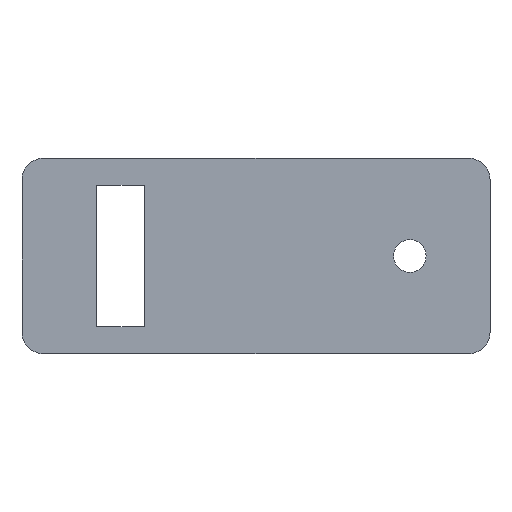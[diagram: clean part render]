
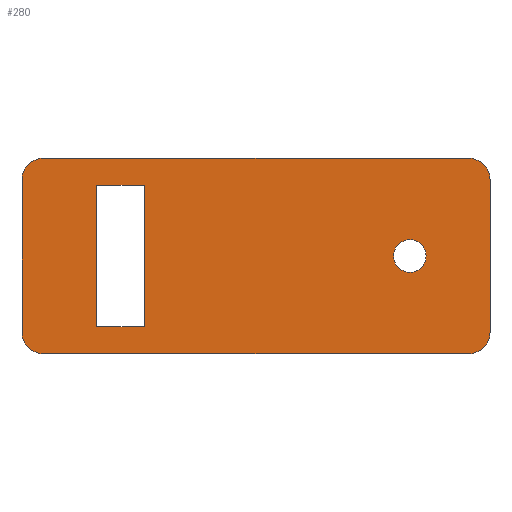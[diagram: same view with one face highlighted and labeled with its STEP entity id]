
A CAD part, top view. The second image highlights one B-rep face of the part: STEP entity #280.
In plain terms, the highlighted planar face has unit normal (0, 0, 1).
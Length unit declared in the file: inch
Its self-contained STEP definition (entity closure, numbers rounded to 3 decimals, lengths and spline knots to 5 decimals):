
#15=FACE_BOUND('',#46,.T.);
#16=FACE_BOUND('',#47,.T.);
#19=PLANE('',#311);
#30=FACE_OUTER_BOUND('',#45,.T.);
#45=EDGE_LOOP('',(#200,#201,#202,#203,#204,#205,#206,#207));
#46=EDGE_LOOP('',(#208,#209,#210,#211));
#47=EDGE_LOOP('',(#212));
#65=LINE('',#426,#94);
#66=LINE('',#430,#95);
#67=LINE('',#434,#96);
#68=LINE('',#437,#97);
#69=LINE('',#440,#98);
#70=LINE('',#442,#99);
#71=LINE('',#444,#100);
#72=LINE('',#445,#101);
#94=VECTOR('',#345,0.3937);
#95=VECTOR('',#348,0.3937);
#96=VECTOR('',#351,0.3937);
#97=VECTOR('',#354,0.3937);
#98=VECTOR('',#355,0.3937);
#99=VECTOR('',#356,0.3937);
#100=VECTOR('',#357,0.3937);
#101=VECTOR('',#358,0.3937);
#121=CIRCLE('',#309,0.11811);
#123=CIRCLE('',#312,0.11811);
#124=CIRCLE('',#313,0.11811);
#125=CIRCLE('',#314,0.11811);
#126=CIRCLE('',#315,0.0885);
#131=VERTEX_POINT('',#416);
#132=VERTEX_POINT('',#417);
#135=VERTEX_POINT('',#425);
#136=VERTEX_POINT('',#427);
#137=VERTEX_POINT('',#429);
#138=VERTEX_POINT('',#431);
#139=VERTEX_POINT('',#433);
#140=VERTEX_POINT('',#435);
#141=VERTEX_POINT('',#438);
#142=VERTEX_POINT('',#439);
#143=VERTEX_POINT('',#441);
#144=VERTEX_POINT('',#443);
#145=VERTEX_POINT('',#446);
#157=EDGE_CURVE('',#131,#132,#121,.T.);
#161=EDGE_CURVE('',#131,#135,#65,.T.);
#162=EDGE_CURVE('',#136,#135,#123,.T.);
#163=EDGE_CURVE('',#137,#136,#66,.T.);
#164=EDGE_CURVE('',#138,#137,#124,.T.);
#165=EDGE_CURVE('',#138,#139,#67,.T.);
#166=EDGE_CURVE('',#140,#139,#125,.T.);
#167=EDGE_CURVE('',#132,#140,#68,.T.);
#168=EDGE_CURVE('',#141,#142,#69,.T.);
#169=EDGE_CURVE('',#143,#141,#70,.T.);
#170=EDGE_CURVE('',#144,#143,#71,.T.);
#171=EDGE_CURVE('',#142,#144,#72,.T.);
#172=EDGE_CURVE('',#145,#145,#126,.T.);
#200=ORIENTED_EDGE('',*,*,#157,.F.);
#201=ORIENTED_EDGE('',*,*,#161,.T.);
#202=ORIENTED_EDGE('',*,*,#162,.F.);
#203=ORIENTED_EDGE('',*,*,#163,.F.);
#204=ORIENTED_EDGE('',*,*,#164,.F.);
#205=ORIENTED_EDGE('',*,*,#165,.T.);
#206=ORIENTED_EDGE('',*,*,#166,.F.);
#207=ORIENTED_EDGE('',*,*,#167,.F.);
#208=ORIENTED_EDGE('',*,*,#168,.F.);
#209=ORIENTED_EDGE('',*,*,#169,.F.);
#210=ORIENTED_EDGE('',*,*,#170,.F.);
#211=ORIENTED_EDGE('',*,*,#171,.F.);
#212=ORIENTED_EDGE('',*,*,#172,.F.);
#280=ADVANCED_FACE('',(#30,#15,#16),#19,.F.);
#309=AXIS2_PLACEMENT_3D('',#418,#337,#338);
#311=AXIS2_PLACEMENT_3D('',#424,#343,#344);
#312=AXIS2_PLACEMENT_3D('',#428,#346,#347);
#313=AXIS2_PLACEMENT_3D('',#432,#349,#350);
#314=AXIS2_PLACEMENT_3D('',#436,#352,#353);
#315=AXIS2_PLACEMENT_3D('',#447,#359,#360);
#337=DIRECTION('center_axis',(0.,0.,
-1.));
#338=DIRECTION('ref_axis',(-0.707,0.707,0.));
#343=DIRECTION('center_axis',(0.,0.,
-1.));
#344=DIRECTION('ref_axis',(1.,0.,0.));
#345=DIRECTION('',(0.,-1.,0.));
#346=DIRECTION('center_axis',(0.,0.,
-1.));
#347=DIRECTION('ref_axis',(-0.707,-0.707,0.));
#348=DIRECTION('',(-1.,0.,0.));
#349=DIRECTION('center_axis',(0.,0.,
-1.));
#350=DIRECTION('ref_axis',(0.707,-0.707,0.));
#351=DIRECTION('',(0.,1.,0.));
#352=DIRECTION('center_axis',(0.,0.,
-1.));
#353=DIRECTION('ref_axis',(0.707,0.707,0.));
#354=DIRECTION('',(1.,0.,0.));
#355=DIRECTION('',(1.,0.,0.));
#356=DIRECTION('',(0.,-1.,0.));
#357=DIRECTION('',(-1.,0.,0.));
#358=DIRECTION('',(0.,1.,0.));
#359=DIRECTION('center_axis',(0.,0.,1.));
#360=DIRECTION('ref_axis',(1.,0.,0.));
#416=CARTESIAN_POINT('',(-11.11339,-1.23228,0.575));
#417=CARTESIAN_POINT('',(-10.99528,-1.11417,0.575));
#418=CARTESIAN_POINT('Origin',(-10.99528,-1.23228,0.575));
#424=CARTESIAN_POINT('Origin',(-9.96919,-1.64665,0.575));
#425=CARTESIAN_POINT('',(-11.11339,-2.06102,0.575));
#426=CARTESIAN_POINT('',(-11.11339,-1.38041,0.575));
#427=CARTESIAN_POINT('',(-10.99528,-2.17913,0.575));
#428=CARTESIAN_POINT('Origin',(-10.99528,-2.06102,0.575));
#429=CARTESIAN_POINT('',(-8.68425,-2.17913,0.575));
#430=CARTESIAN_POINT('',(-8.64921,-2.17913,0.575));
#431=CARTESIAN_POINT('',(-8.56614,-2.06102,0.575));
#432=CARTESIAN_POINT('Origin',(-8.68425,-2.06102,0.575));
#433=CARTESIAN_POINT('',(-8.56614,-1.23228,0.575));
#434=CARTESIAN_POINT('',(-8.56614,-2.17913,0.575));
#435=CARTESIAN_POINT('',(-8.68425,-1.11417,0.575));
#436=CARTESIAN_POINT('Origin',(-8.68425,-1.23228,0.575));
#437=CARTESIAN_POINT('',(-11.28917,-1.11417,0.575));
#438=CARTESIAN_POINT('',(-10.70787,-2.0315,0.575));
#439=CARTESIAN_POINT('',(-10.44685,-2.0315,0.575));
#440=CARTESIAN_POINT('',(-10.70787,-2.0315,0.575));
#441=CARTESIAN_POINT('',(-10.70787,-1.26181,0.575));
#442=CARTESIAN_POINT('',(-10.70787,-1.67927,0.575));
#443=CARTESIAN_POINT('',(-10.44685,-1.26181,0.575));
#444=CARTESIAN_POINT('',(-10.44685,-1.26181,0.575));
#445=CARTESIAN_POINT('',(-10.44685,-1.61404,0.575));
#446=CARTESIAN_POINT('',(-9.09086,-1.64665,0.575));
#447=CARTESIAN_POINT('Origin',(-9.00236,-1.64665,0.575));
